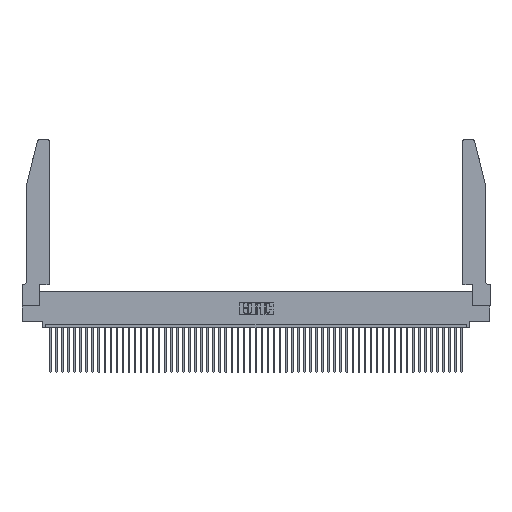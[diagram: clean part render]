
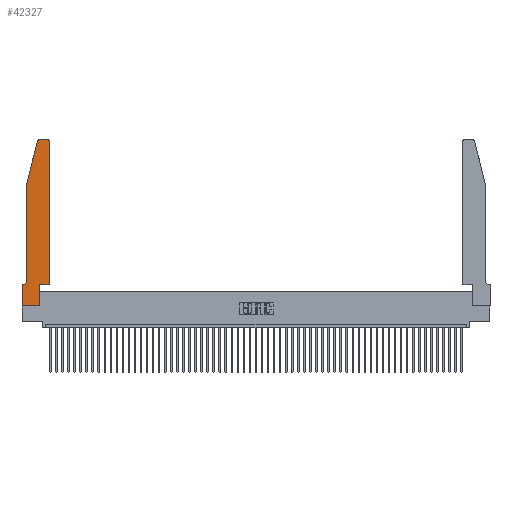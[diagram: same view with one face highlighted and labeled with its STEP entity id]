
A CAD part, top view. The second image highlights one B-rep face of the part: STEP entity #42327.
In plain terms, the highlighted planar face has unit normal (0, 0, 1).
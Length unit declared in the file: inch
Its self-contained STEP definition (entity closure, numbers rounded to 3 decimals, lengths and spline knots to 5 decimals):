
#1751 = AXIS2_PLACEMENT_3D ( 'NONE', #51641, #35688, #23846 ) ;
#1844 = DIRECTION ( 'NONE',  ( 0., 1., 0. ) ) ;
#2524 = VECTOR ( 'NONE', #22694, 39.37008 ) ;
#2953 = ORIENTED_EDGE ( 'NONE', *, *, #25477, .T. ) ;
#3202 = VERTEX_POINT ( 'NONE', #32162 ) ;
#3406 = LINE ( 'NONE', #10755, #38656 ) ;
#3441 = DIRECTION ( 'NONE',  ( 0., -1., 0. ) ) ;
#3528 = CARTESIAN_POINT ( 'NONE',  ( 0.0755, 2., 0.37 ) ) ;
#3834 = VECTOR ( 'NONE', #50577, 39.37008 ) ;
#4258 = ORIENTED_EDGE ( 'NONE', *, *, #8393, .T. ) ;
#4280 = CARTESIAN_POINT ( 'NONE',  ( 0., 0.35, 0.37 ) ) ;
#5193 = CARTESIAN_POINT ( 'NONE',  ( 0.4205, 2.75, 0.37 ) ) ;
#5377 = VERTEX_POINT ( 'NONE', #27771 ) ;
#5463 = PLANE ( 'NONE',  #28458 ) ;
#5774 = LINE ( 'NONE', #38247, #44369 ) ;
#5863 = ORIENTED_EDGE ( 'NONE', *, *, #52828, .T. ) ;
#6062 = ORIENTED_EDGE ( 'NONE', *, *, #48517, .T. ) ;
#6141 = VERTEX_POINT ( 'NONE', #3528 ) ;
#6771 = CARTESIAN_POINT ( 'NONE',  ( 0.2865, 0.35, 0.37 ) ) ;
#6846 = ORIENTED_EDGE ( 'NONE', *, *, #26857, .T. ) ;
#6907 = DIRECTION ( 'NONE',  ( -1., 0., 0. ) ) ;
#8153 = AXIS2_PLACEMENT_3D ( 'NONE', #19090, #27894, #6907 ) ;
#8393 = EDGE_CURVE ( 'NONE', #3202, #6141, #9370, .T. ) ;
#8410 = ORIENTED_EDGE ( 'NONE', *, *, #11653, .T. ) ;
#9370 = LINE ( 'NONE', #31994, #34425 ) ;
#9910 = CARTESIAN_POINT ( 'NONE',  ( 0.0755, 0.42, 0.37 ) ) ;
#10755 = CARTESIAN_POINT ( 'NONE',  ( 0.2865, 0.35, 0.37 ) ) ;
#10777 = CARTESIAN_POINT ( 'NONE',  ( 0.4205, 2.72, 0.37 ) ) ;
#11153 = ORIENTED_EDGE ( 'NONE', *, *, #41694, .T. ) ;
#11307 = CARTESIAN_POINT ( 'NONE',  ( 0., 0., 0.37 ) ) ;
#11653 = EDGE_CURVE ( 'NONE', #18847, #33201, #26134, .T. ) ;
#12476 = CARTESIAN_POINT ( 'NONE',  ( 0., 0., 0.37 ) ) ;
#12675 = EDGE_CURVE ( 'NONE', #18488, #40213, #33719, .T. ) ;
#14455 = VECTOR ( 'NONE', #3441, 39.37008 ) ;
#15363 = VECTOR ( 'NONE', #48552, 39.37008 ) ;
#15565 = CARTESIAN_POINT ( 'NONE',  ( 0.4505, 0.35, 0.37 ) ) ;
#17499 = ORIENTED_EDGE ( 'NONE', *, *, #17951, .T. ) ;
#17951 = EDGE_CURVE ( 'NONE', #36367, #40414, #25530, .T. ) ;
#18488 = VERTEX_POINT ( 'NONE', #9910 ) ;
#18847 = VERTEX_POINT ( 'NONE', #6771 ) ;
#19090 = CARTESIAN_POINT ( 'NONE',  ( 0.0055, 0.42, 0.37 ) ) ;
#21102 = LINE ( 'NONE', #11307, #22382 ) ;
#21516 = LINE ( 'NONE', #23514, #14455 ) ;
#22382 = VECTOR ( 'NONE', #26875, 39.37008 ) ;
#22525 = DIRECTION ( 'NONE',  ( 0., 0., 1. ) ) ;
#22684 = ORIENTED_EDGE ( 'NONE', *, *, #38834, .T. ) ;
#22694 = DIRECTION ( 'NONE',  ( 0., 1., 0. ) ) ;
#22812 = ORIENTED_EDGE ( 'NONE', *, *, #12675, .T. ) ;
#23186 = EDGE_CURVE ( 'NONE', #40414, #3202, #44646, .T. ) ;
#23514 = CARTESIAN_POINT ( 'NONE',  ( 0., 0., 0.37 ) ) ;
#23846 = DIRECTION ( 'NONE',  ( 1., 0., 0. ) ) ;
#24087 = DIRECTION ( 'NONE',  ( -0.239, -0.971, 0. ) ) ;
#25477 = EDGE_CURVE ( 'NONE', #5377, #36367, #52182, .T. ) ;
#25530 = LINE ( 'NONE', #29103, #3834 ) ;
#26134 = LINE ( 'NONE', #15565, #15363 ) ;
#26502 = DIRECTION ( 'NONE',  ( 0., -1., 0. ) ) ;
#26857 = EDGE_CURVE ( 'NONE', #33201, #5377, #46118, .T. ) ;
#26875 = DIRECTION ( 'NONE',  ( 1., 0., 0. ) ) ;
#27771 = CARTESIAN_POINT ( 'NONE',  ( 0.4505, 2.72, 0.37 ) ) ;
#27812 = CARTESIAN_POINT ( 'NONE',  ( 0.2865, 0., 0.37 ) ) ;
#27894 = DIRECTION ( 'NONE',  ( 0., 0., -1. ) ) ;
#28458 = AXIS2_PLACEMENT_3D ( 'NONE', #30812, #22525, #42613 ) ;
#28655 = ORIENTED_EDGE ( 'NONE', *, *, #32557, .T. ) ;
#29103 = CARTESIAN_POINT ( 'NONE',  ( 0.2605, 2.75, 0.37 ) ) ;
#30812 = CARTESIAN_POINT ( 'NONE',  ( 0., 0.35, 0.37 ) ) ;
#31055 = CARTESIAN_POINT ( 'NONE',  ( 0.4505, 0.35, 0.37 ) ) ;
#31443 = DIRECTION ( 'NONE',  ( 1., 0., 0. ) ) ;
#31478 = VECTOR ( 'NONE', #26502, 39.37008 ) ;
#31994 = CARTESIAN_POINT ( 'NONE',  ( 0.0755, 2., 0.37 ) ) ;
#32162 = CARTESIAN_POINT ( 'NONE',  ( 0.25487, 2.72718, 0.37 ) ) ;
#32557 = EDGE_CURVE ( 'NONE', #6141, #18488, #42278, .T. ) ;
#33201 = VERTEX_POINT ( 'NONE', #31055 ) ;
#33719 = CIRCLE ( 'NONE', #8153, 0.07 ) ;
#34425 = VECTOR ( 'NONE', #24087, 39.37008 ) ;
#34964 = CARTESIAN_POINT ( 'NONE',  ( 0.0755, 2., 0.37 ) ) ;
#35685 = CARTESIAN_POINT ( 'NONE',  ( 0.4505, 0.35, 0.37 ) ) ;
#35688 = DIRECTION ( 'NONE',  ( 0., 0., 1. ) ) ;
#36367 = VERTEX_POINT ( 'NONE', #5193 ) ;
#38247 = CARTESIAN_POINT ( 'NONE',  ( 0.0755, 0.35, 0.37 ) ) ;
#38656 = VECTOR ( 'NONE', #1844, 39.37008 ) ;
#38834 = EDGE_CURVE ( 'NONE', #40213, #53078, #5774, .T. ) ;
#39516 = DIRECTION ( 'NONE',  ( 0., 0., 1. ) ) ;
#40213 = VERTEX_POINT ( 'NONE', #46368 ) ;
#40414 = VERTEX_POINT ( 'NONE', #50614 ) ;
#41308 = AXIS2_PLACEMENT_3D ( 'NONE', #10777, #39516, #31443 ) ;
#41694 = EDGE_CURVE ( 'NONE', #53078, #42711, #21516, .T. ) ;
#42278 = LINE ( 'NONE', #34964, #31478 ) ;
#42327 = ADVANCED_FACE ( 'NONE', ( #47689 ), #5463, .T. ) ;
#42613 = DIRECTION ( 'NONE',  ( 1., 0., 0. ) ) ;
#42711 = VERTEX_POINT ( 'NONE', #12476 ) ;
#42912 = ORIENTED_EDGE ( 'NONE', *, *, #23186, .T. ) ;
#44369 = VECTOR ( 'NONE', #51571, 39.37008 ) ;
#44379 = VERTEX_POINT ( 'NONE', #27812 ) ;
#44646 = CIRCLE ( 'NONE', #1751, 0.03 ) ;
#46118 = LINE ( 'NONE', #35685, #2524 ) ;
#46368 = CARTESIAN_POINT ( 'NONE',  ( 0.0055, 0.35, 0.37 ) ) ;
#47689 = FACE_OUTER_BOUND ( 'NONE', #52083, .T. ) ;
#48517 = EDGE_CURVE ( 'NONE', #42711, #44379, #21102, .T. ) ;
#48552 = DIRECTION ( 'NONE',  ( 1., 0., 0. ) ) ;
#50577 = DIRECTION ( 'NONE',  ( -1., 0., 0. ) ) ;
#50614 = CARTESIAN_POINT ( 'NONE',  ( 0.284, 2.75, 0.37 ) ) ;
#51571 = DIRECTION ( 'NONE',  ( -1., 0., 0. ) ) ;
#51641 = CARTESIAN_POINT ( 'NONE',  ( 0.284, 2.72, 0.37 ) ) ;
#52083 = EDGE_LOOP ( 'NONE', ( #17499, #42912, #4258, #28655, #22812, #22684, #11153, #6062, #5863, #8410, #6846, #2953 ) ) ;
#52182 = CIRCLE ( 'NONE', #41308, 0.03 ) ;
#52828 = EDGE_CURVE ( 'NONE', #44379, #18847, #3406, .T. ) ;
#53078 = VERTEX_POINT ( 'NONE', #4280 ) ;
